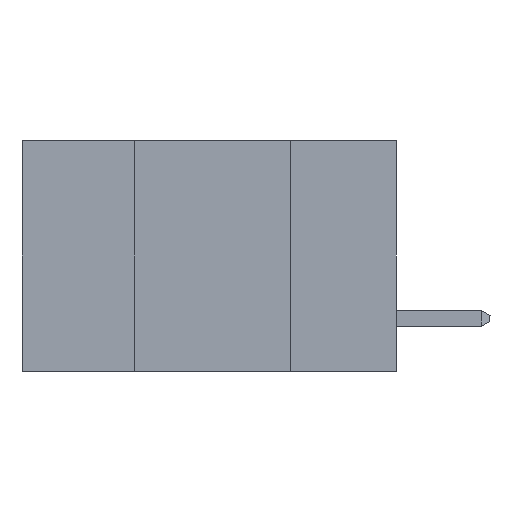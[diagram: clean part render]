
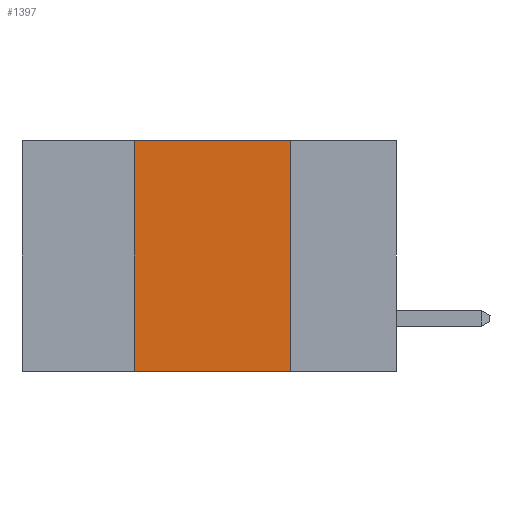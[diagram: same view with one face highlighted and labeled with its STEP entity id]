
A CAD part, left-side view. The second image highlights one B-rep face of the part: STEP entity #1397.
In plain terms, the highlighted planar face has unit normal (-1, 0, 0).
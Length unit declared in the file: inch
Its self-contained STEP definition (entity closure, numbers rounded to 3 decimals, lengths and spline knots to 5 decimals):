
#60 = CARTESIAN_POINT ( 'NONE',  ( 0., 0.42, 0. ) ) ;
#75 = PLANE ( 'NONE',  #10379 ) ;
#309 = EDGE_CURVE ( 'NONE', #2941, #1347, #4993, .T. ) ;
#328 = CARTESIAN_POINT ( 'NONE',  ( 0., 0.6, -0.37 ) ) ;
#694 = CARTESIAN_POINT ( 'NONE',  ( 0., 0.6, 0. ) ) ;
#1033 = ORIENTED_EDGE ( 'NONE', *, *, #3972, .F. ) ;
#1347 = VERTEX_POINT ( 'NONE', #9648 ) ;
#1397 = ADVANCED_FACE ( 'NONE', ( #7828 ), #75, .F. ) ;
#2518 = ORIENTED_EDGE ( 'NONE', *, *, #309, .T. ) ;
#2761 = VECTOR ( 'NONE', #8432, 39.37008 ) ;
#2941 = VERTEX_POINT ( 'NONE', #8226 ) ;
#3151 = CARTESIAN_POINT ( 'NONE',  ( 0., 0.42, -0.37 ) ) ;
#3714 = VERTEX_POINT ( 'NONE', #60 ) ;
#3972 = EDGE_CURVE ( 'NONE', #3714, #7106, #7843, .T. ) ;
#4177 = CARTESIAN_POINT ( 'NONE',  ( 0., 0.17, -0.37 ) ) ;
#4330 = EDGE_CURVE ( 'NONE', #7106, #1347, #9061, .T. ) ;
#4993 = LINE ( 'NONE', #328, #2761 ) ;
#5624 = VECTOR ( 'NONE', #9446, 39.37008 ) ;
#6100 = ORIENTED_EDGE ( 'NONE', *, *, #8083, .F. ) ;
#6212 = CARTESIAN_POINT ( 'NONE',  ( 0., 0.6, 0. ) ) ;
#6504 = CARTESIAN_POINT ( 'NONE',  ( 0., 0.17, 0. ) ) ;
#6678 = VECTOR ( 'NONE', #8273, 39.37008 ) ;
#7001 = ORIENTED_EDGE ( 'NONE', *, *, #4330, .F. ) ;
#7106 = VERTEX_POINT ( 'NONE', #6504 ) ;
#7115 = VECTOR ( 'NONE', #10486, 39.37008 ) ;
#7828 = FACE_OUTER_BOUND ( 'NONE', #8062, .T. ) ;
#7843 = LINE ( 'NONE', #6212, #5624 ) ;
#8062 = EDGE_LOOP ( 'NONE', ( #7001, #1033, #6100, #2518 ) ) ;
#8083 = EDGE_CURVE ( 'NONE', #2941, #3714, #9244, .T. ) ;
#8226 = CARTESIAN_POINT ( 'NONE',  ( 0., 0.42, -0.37 ) ) ;
#8273 = DIRECTION ( 'NONE',  ( 0., 0., -1. ) ) ;
#8432 = DIRECTION ( 'NONE',  ( 0., -1., 0. ) ) ;
#9061 = LINE ( 'NONE', #4177, #6678 ) ;
#9244 = LINE ( 'NONE', #3151, #7115 ) ;
#9281 = DIRECTION ( 'NONE',  ( 0., 0., -1. ) ) ;
#9446 = DIRECTION ( 'NONE',  ( 0., -1., 0. ) ) ;
#9648 = CARTESIAN_POINT ( 'NONE',  ( 0., 0.17, -0.37 ) ) ;
#9810 = DIRECTION ( 'NONE',  ( 1., 0., 0. ) ) ;
#10379 = AXIS2_PLACEMENT_3D ( 'NONE', #694, #9810, #9281 ) ;
#10486 = DIRECTION ( 'NONE',  ( 0., 0., 1. ) ) ;
